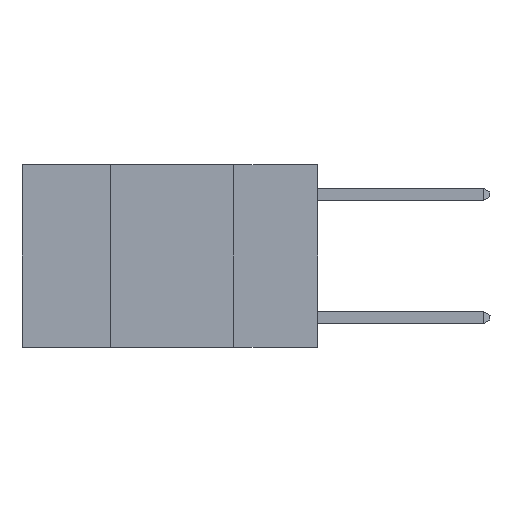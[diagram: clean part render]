
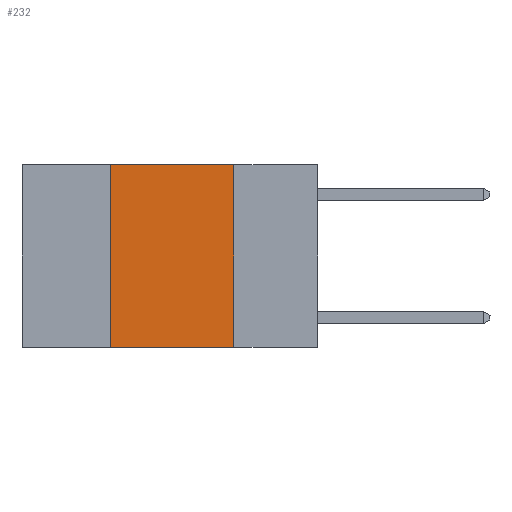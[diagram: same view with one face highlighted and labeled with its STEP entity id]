
A CAD part, left-side view. The second image highlights one B-rep face of the part: STEP entity #232.
In plain terms, the highlighted planar face has unit normal (-1, 0, 0).
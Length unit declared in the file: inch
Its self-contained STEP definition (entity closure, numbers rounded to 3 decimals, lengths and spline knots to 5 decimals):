
#232 = ADVANCED_FACE ( 'NONE', ( #13402 ), #15520, .F. ) ;
#650 = CARTESIAN_POINT ( 'NONE',  ( 0., 0.17, -0.37 ) ) ;
#1950 = EDGE_CURVE ( 'NONE', #9631, #7442, #17467, .T. ) ;
#2788 = DIRECTION ( 'NONE',  ( 0., 0., 1. ) ) ;
#3181 = CARTESIAN_POINT ( 'NONE',  ( 0., 0.42, 0. ) ) ;
#6193 = VERTEX_POINT ( 'NONE', #6305 ) ;
#6305 = CARTESIAN_POINT ( 'NONE',  ( 0., 0.17, 0. ) ) ;
#6504 = EDGE_CURVE ( 'NONE', #9631, #12150, #11200, .T. ) ;
#6646 = DIRECTION ( 'NONE',  ( 1., 0., 0. ) ) ;
#7010 = AXIS2_PLACEMENT_3D ( 'NONE', #9552, #6646, #9315 ) ;
#7085 = ORIENTED_EDGE ( 'NONE', *, *, #6504, .T. ) ;
#7215 = VECTOR ( 'NONE', #7610, 39.37008 ) ;
#7442 = VERTEX_POINT ( 'NONE', #16646 ) ;
#7463 = VECTOR ( 'NONE', #15637, 39.37008 ) ;
#7610 = DIRECTION ( 'NONE',  ( 0., -1., 0. ) ) ;
#7912 = LINE ( 'NONE', #14276, #7463 ) ;
#9315 = DIRECTION ( 'NONE',  ( 0., 0., -1. ) ) ;
#9552 = CARTESIAN_POINT ( 'NONE',  ( 0., 0.6, 0. ) ) ;
#9631 = VERTEX_POINT ( 'NONE', #10400 ) ;
#10400 = CARTESIAN_POINT ( 'NONE',  ( 0., 0.42, -0.37 ) ) ;
#10546 = EDGE_LOOP ( 'NONE', ( #12348, #13390, #13385, #7085 ) ) ;
#10626 = LINE ( 'NONE', #14264, #17270 ) ;
#11200 = LINE ( 'NONE', #12915, #7215 ) ;
#12150 = VERTEX_POINT ( 'NONE', #650 ) ;
#12348 = ORIENTED_EDGE ( 'NONE', *, *, #14210, .F. ) ;
#12915 = CARTESIAN_POINT ( 'NONE',  ( 0., 0.6, -0.37 ) ) ;
#13385 = ORIENTED_EDGE ( 'NONE', *, *, #1950, .F. ) ;
#13390 = ORIENTED_EDGE ( 'NONE', *, *, #16560, .F. ) ;
#13402 = FACE_OUTER_BOUND ( 'NONE', #10546, .T. ) ;
#13935 = VECTOR ( 'NONE', #2788, 39.37008 ) ;
#14210 = EDGE_CURVE ( 'NONE', #6193, #12150, #10626, .T. ) ;
#14264 = CARTESIAN_POINT ( 'NONE',  ( 0., 0.17, 0. ) ) ;
#14276 = CARTESIAN_POINT ( 'NONE',  ( 0., 0.6, 0. ) ) ;
#15520 = PLANE ( 'NONE',  #7010 ) ;
#15628 = DIRECTION ( 'NONE',  ( 0., 0., -1. ) ) ;
#15637 = DIRECTION ( 'NONE',  ( 0., -1., 0. ) ) ;
#16560 = EDGE_CURVE ( 'NONE', #7442, #6193, #7912, .T. ) ;
#16646 = CARTESIAN_POINT ( 'NONE',  ( 0., 0.42, 0. ) ) ;
#17270 = VECTOR ( 'NONE', #15628, 39.37008 ) ;
#17467 = LINE ( 'NONE', #3181, #13935 ) ;
